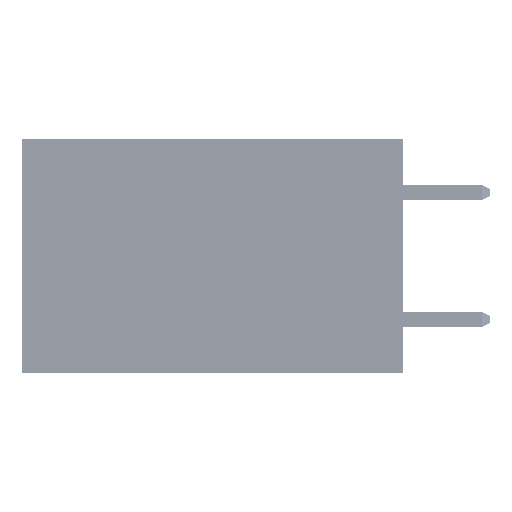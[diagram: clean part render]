
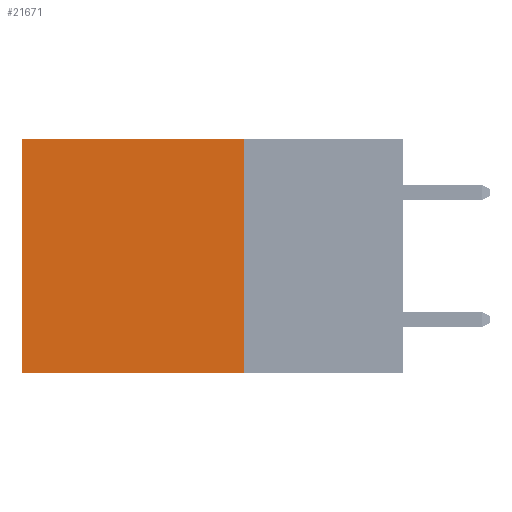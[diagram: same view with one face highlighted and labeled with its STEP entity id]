
A CAD part, left-side view. The second image highlights one B-rep face of the part: STEP entity #21671.
In plain terms, the highlighted planar face has unit normal (-1, 0, 0).
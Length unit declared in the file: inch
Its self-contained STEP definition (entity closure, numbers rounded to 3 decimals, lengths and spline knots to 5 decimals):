
#40 = CARTESIAN_POINT ( 'NONE',  ( 0.2875, 0.25, 0. ) ) ;
#1110 = VECTOR ( 'NONE', #12793, 39.37008 ) ;
#3260 = DIRECTION ( 'NONE',  ( 0., 0., -1. ) ) ;
#3294 = CARTESIAN_POINT ( 'NONE',  ( 0.2875, 0.25, 0. ) ) ;
#4062 = LINE ( 'NONE', #7240, #41700 ) ;
#7240 = CARTESIAN_POINT ( 'NONE',  ( 0.2875, 0.6, 0. ) ) ;
#7348 = ORIENTED_EDGE ( 'NONE', *, *, #39669, .F. ) ;
#10862 = DIRECTION ( 'NONE',  ( 0., 0., -1. ) ) ;
#10872 = VECTOR ( 'NONE', #18258, 39.37008 ) ;
#11256 = VECTOR ( 'NONE', #3260, 39.37008 ) ;
#12793 = DIRECTION ( 'NONE',  ( 0., 1., 0. ) ) ;
#17683 = CARTESIAN_POINT ( 'NONE',  ( 0.2875, 0.6, -0.37 ) ) ;
#18258 = DIRECTION ( 'NONE',  ( 0., 1., 0. ) ) ;
#18486 = FACE_OUTER_BOUND ( 'NONE', #21737, .T. ) ;
#20482 = ORIENTED_EDGE ( 'NONE', *, *, #30337, .T. ) ;
#20706 = ORIENTED_EDGE ( 'NONE', *, *, #23441, .T. ) ;
#20868 = CARTESIAN_POINT ( 'NONE',  ( 0.2875, 0.25, -0.37 ) ) ;
#21671 = ADVANCED_FACE ( 'NONE', ( #18486 ), #21912, .F. ) ;
#21737 = EDGE_LOOP ( 'NONE', ( #20706, #38595, #7348, #20482 ) ) ;
#21912 = PLANE ( 'NONE',  #46968 ) ;
#23441 = EDGE_CURVE ( 'NONE', #44351, #26696, #4062, .T. ) ;
#23933 = VERTEX_POINT ( 'NONE', #34071 ) ;
#26341 = CARTESIAN_POINT ( 'NONE',  ( 0.2875, 0.6, 0. ) ) ;
#26696 = VERTEX_POINT ( 'NONE', #17683 ) ;
#29714 = LINE ( 'NONE', #40, #11256 ) ;
#30337 = EDGE_CURVE ( 'NONE', #23933, #44351, #32965, .T. ) ;
#32428 = VERTEX_POINT ( 'NONE', #20868 ) ;
#32965 = LINE ( 'NONE', #37094, #10872 ) ;
#34071 = CARTESIAN_POINT ( 'NONE',  ( 0.2875, 0.25, 0. ) ) ;
#34612 = LINE ( 'NONE', #38759, #1110 ) ;
#37094 = CARTESIAN_POINT ( 'NONE',  ( 0.2875, 0.25, 0. ) ) ;
#37968 = EDGE_CURVE ( 'NONE', #32428, #26696, #34612, .T. ) ;
#38595 = ORIENTED_EDGE ( 'NONE', *, *, #37968, .F. ) ;
#38759 = CARTESIAN_POINT ( 'NONE',  ( 0.2875, 0.25, -0.37 ) ) ;
#39669 = EDGE_CURVE ( 'NONE', #23933, #32428, #29714, .T. ) ;
#41700 = VECTOR ( 'NONE', #42943, 39.37008 ) ;
#42943 = DIRECTION ( 'NONE',  ( 0., 0., -1. ) ) ;
#44351 = VERTEX_POINT ( 'NONE', #26341 ) ;
#44410 = DIRECTION ( 'NONE',  ( 1., 0., 0. ) ) ;
#46968 = AXIS2_PLACEMENT_3D ( 'NONE', #3294, #44410, #10862 ) ;
